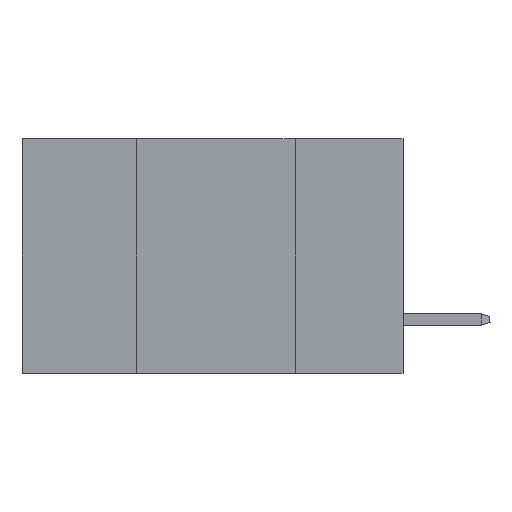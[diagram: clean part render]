
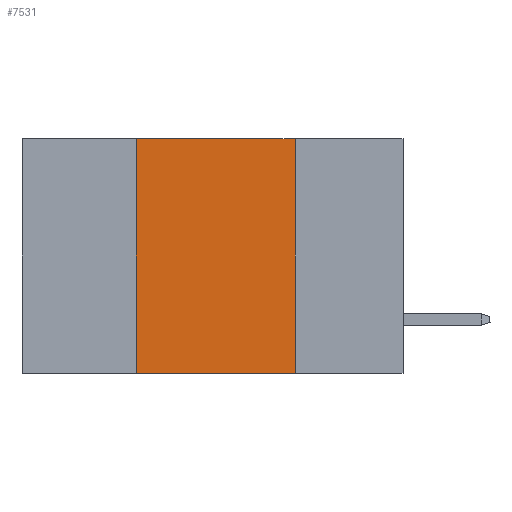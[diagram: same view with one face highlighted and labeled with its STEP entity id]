
A CAD part, left-side view. The second image highlights one B-rep face of the part: STEP entity #7531.
In plain terms, the highlighted planar face has unit normal (-1, 0, 0).
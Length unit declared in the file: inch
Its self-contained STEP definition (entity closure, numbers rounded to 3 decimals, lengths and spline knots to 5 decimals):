
#277 = CARTESIAN_POINT ( 'NONE',  ( 0., 0.6, -0.37 ) ) ;
#831 = ORIENTED_EDGE ( 'NONE', *, *, #3415, .F. ) ;
#2074 = ORIENTED_EDGE ( 'NONE', *, *, #25527, .F. ) ;
#3413 = CARTESIAN_POINT ( 'NONE',  ( 0., 0.6, 0. ) ) ;
#3415 = EDGE_CURVE ( 'NONE', #6812, #19478, #13385, .T. ) ;
#3568 = VERTEX_POINT ( 'NONE', #4028 ) ;
#4028 = CARTESIAN_POINT ( 'NONE',  ( 0., 0.17, -0.37 ) ) ;
#4146 = ORIENTED_EDGE ( 'NONE', *, *, #13185, .F. ) ;
#4715 = VERTEX_POINT ( 'NONE', #8573 ) ;
#6647 = ORIENTED_EDGE ( 'NONE', *, *, #17823, .T. ) ;
#6812 = VERTEX_POINT ( 'NONE', #18072 ) ;
#7531 = ADVANCED_FACE ( 'NONE', ( #17480 ), #11276, .F. ) ;
#7957 = DIRECTION ( 'NONE',  ( 0., 0., 1. ) ) ;
#8573 = CARTESIAN_POINT ( 'NONE',  ( 0., 0.42, -0.37 ) ) ;
#8786 = DIRECTION ( 'NONE',  ( 0., 0., -1. ) ) ;
#9038 = VECTOR ( 'NONE', #15691, 39.37008 ) ;
#10954 = DIRECTION ( 'NONE',  ( 0., -1., 0. ) ) ;
#11276 = PLANE ( 'NONE',  #19945 ) ;
#12846 = EDGE_LOOP ( 'NONE', ( #4146, #831, #2074, #6647 ) ) ;
#12884 = VECTOR ( 'NONE', #8786, 39.37008 ) ;
#13185 = EDGE_CURVE ( 'NONE', #19478, #3568, #14909, .T. ) ;
#13358 = DIRECTION ( 'NONE',  ( 1., 0., 0. ) ) ;
#13385 = LINE ( 'NONE', #3413, #9038 ) ;
#14909 = LINE ( 'NONE', #18646, #12884 ) ;
#15665 = DIRECTION ( 'NONE',  ( 0., 0., -1. ) ) ;
#15691 = DIRECTION ( 'NONE',  ( 0., -1., 0. ) ) ;
#15861 = LINE ( 'NONE', #17927, #21838 ) ;
#17480 = FACE_OUTER_BOUND ( 'NONE', #12846, .T. ) ;
#17823 = EDGE_CURVE ( 'NONE', #4715, #3568, #20684, .T. ) ;
#17927 = CARTESIAN_POINT ( 'NONE',  ( 0., 0.42, 0. ) ) ;
#18072 = CARTESIAN_POINT ( 'NONE',  ( 0., 0.42, 0. ) ) ;
#18646 = CARTESIAN_POINT ( 'NONE',  ( 0., 0.17, 0. ) ) ;
#19478 = VERTEX_POINT ( 'NONE', #21992 ) ;
#19918 = VECTOR ( 'NONE', #10954, 39.37008 ) ;
#19945 = AXIS2_PLACEMENT_3D ( 'NONE', #23346, #13358, #15665 ) ;
#20684 = LINE ( 'NONE', #277, #19918 ) ;
#21838 = VECTOR ( 'NONE', #7957, 39.37008 ) ;
#21992 = CARTESIAN_POINT ( 'NONE',  ( 0., 0.17, 0. ) ) ;
#23346 = CARTESIAN_POINT ( 'NONE',  ( 0., 0.6, 0. ) ) ;
#25527 = EDGE_CURVE ( 'NONE', #4715, #6812, #15861, .T. ) ;
